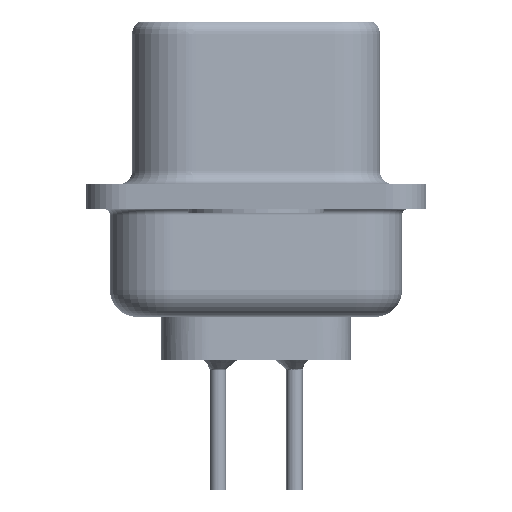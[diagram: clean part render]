
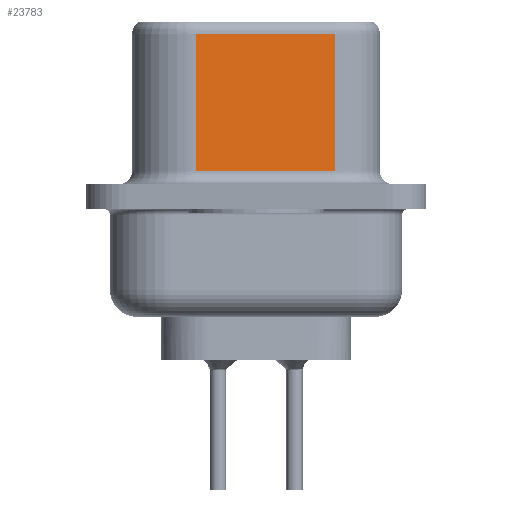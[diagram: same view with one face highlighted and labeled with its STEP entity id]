
A CAD part, left-side view. The second image highlights one B-rep face of the part: STEP entity #23783.
In plain terms, the highlighted planar face has unit normal (-0.985, -0.174, 0).
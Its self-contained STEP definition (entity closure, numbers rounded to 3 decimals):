
#1078 = VECTOR ( 'NONE', #19021, 1000. ) ;
#2305 = VERTEX_POINT ( 'NONE', #5348 ) ;
#3138 = EDGE_CURVE ( 'NONE', #16614, #2305, #9930, .T. ) ;
#3785 = DIRECTION ( 'NONE',  ( 0., 0., -1. ) ) ;
#5348 = CARTESIAN_POINT ( 'NONE',  ( 3.67, 2.233, 0.95 ) ) ;
#5366 = VECTOR ( 'NONE', #3785, 1000. ) ;
#5382 = VECTOR ( 'NONE', #23271, 1000. ) ;
#7002 = EDGE_CURVE ( 'NONE', #2305, #16859, #22708, .T. ) ;
#7867 = DIRECTION ( 'NONE',  ( -0.174, 0.985, 0. ) ) ;
#8147 = CARTESIAN_POINT ( 'NONE',  ( 3.67, 2.233, 6.02 ) ) ;
#9616 = ORIENTED_EDGE ( 'NONE', *, *, #16373, .T. ) ;
#9930 = LINE ( 'NONE', #12721, #1078 ) ;
#10167 = AXIS2_PLACEMENT_3D ( 'NONE', #22724, #20209, #20630 ) ;
#10207 = LINE ( 'NONE', #14670, #5366 ) ;
#11450 = EDGE_CURVE ( 'NONE', #12976, #16859, #10207, .T. ) ;
#11741 = ORIENTED_EDGE ( 'NONE', *, *, #3138, .T. ) ;
#12550 = CARTESIAN_POINT ( 'NONE',  ( 4.58, -2.927, 0.95 ) ) ;
#12721 = CARTESIAN_POINT ( 'NONE',  ( 3.67, 2.233, 6.52 ) ) ;
#12976 = VERTEX_POINT ( 'NONE', #17890 ) ;
#14062 = PLANE ( 'NONE',  #10167 ) ;
#14670 = CARTESIAN_POINT ( 'NONE',  ( 4.58, -2.927, 6.52 ) ) ;
#16295 = FACE_OUTER_BOUND ( 'NONE', #19273, .T. ) ;
#16373 = EDGE_CURVE ( 'NONE', #12976, #16614, #22414, .T. ) ;
#16614 = VERTEX_POINT ( 'NONE', #8147 ) ;
#16859 = VERTEX_POINT ( 'NONE', #12550 ) ;
#17890 = CARTESIAN_POINT ( 'NONE',  ( 4.58, -2.927, 6.02 ) ) ;
#19021 = DIRECTION ( 'NONE',  ( 0., 0., -1. ) ) ;
#19273 = EDGE_LOOP ( 'NONE', ( #22825, #9616, #11741, #26097 ) ) ;
#20209 = DIRECTION ( 'NONE',  ( 0.985, 0.174, 0. ) ) ;
#20448 = CARTESIAN_POINT ( 'NONE',  ( 4.58, -2.927, 6.02 ) ) ;
#20630 = DIRECTION ( 'NONE',  ( -0.174, 0.985, 0. ) ) ;
#20734 = VECTOR ( 'NONE', #7867, 1000. ) ;
#22414 = LINE ( 'NONE', #20448, #20734 ) ;
#22708 = LINE ( 'NONE', #25108, #5382 ) ;
#22724 = CARTESIAN_POINT ( 'NONE',  ( 4.58, -2.927, 6.52 ) ) ;
#22825 = ORIENTED_EDGE ( 'NONE', *, *, #11450, .F. ) ;
#23271 = DIRECTION ( 'NONE',  ( 0.174, -0.985, 0. ) ) ;
#23783 = ADVANCED_FACE ( 'NONE', ( #16295 ), #14062, .F. ) ;
#25108 = CARTESIAN_POINT ( 'NONE',  ( 4.58, -2.927, 0.95 ) ) ;
#26097 = ORIENTED_EDGE ( 'NONE', *, *, #7002, .T. ) ;
